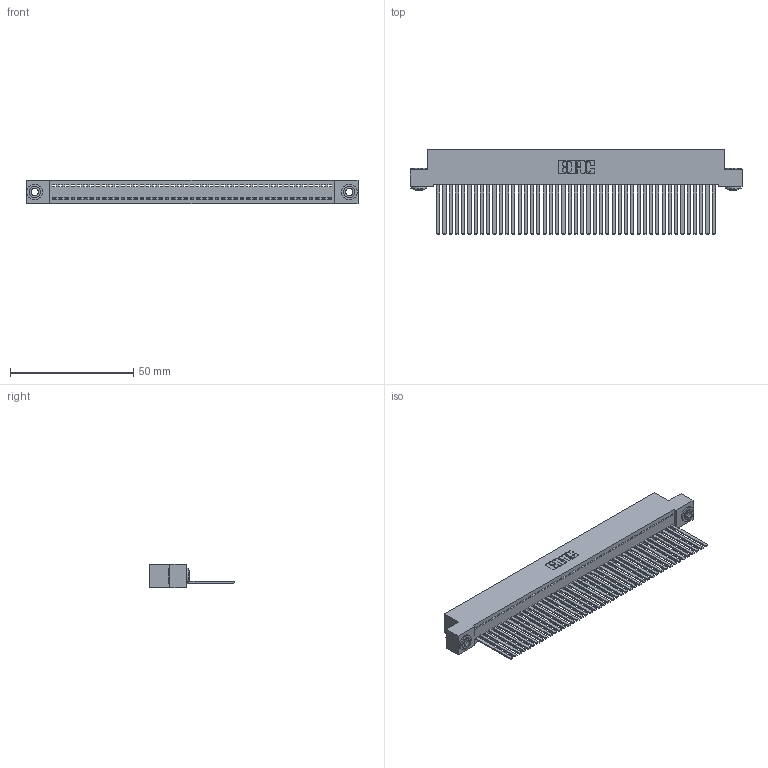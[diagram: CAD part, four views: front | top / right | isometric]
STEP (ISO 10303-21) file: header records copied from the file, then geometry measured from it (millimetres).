
FILE_DESCRIPTION (( 'STEP AP203' ), '1' );
FILE_NAME ('342-045-544-103.STEP', '2018-08-12T15:32:29', ( '' ), ( '' ), 'SwSTEP 2.0', 'SolidWorks 2016', '' );
FILE_SCHEMA (( 'CONFIG_CONTROL_DESIGN' ));
Length unit declared in the file: inch
Products named in the file (4): 342 Part_.156 TH; 345-292-001_345-293-144; 342-250-002_345-250-002-102; 342-045-544-103
Assembly tree (48 placements, depth 2):
  342-045-544-103
    342 Part_.156 TH
    345-292-001_345-293-144  x45
    342-250-002_345-250-002-102  x2
Bounding box: 134.62 x 34.3 x 9.4 mm (x, y, z)
Volume: 12358.5 mm3; surface area: 19913.4 mm2
Topology: 48 solids, 48 shells, 2488 faces, 7485 edges, 4926 vertices
Faces by surface type: plane 1786, cylinder 694, cone 8
Entity records: 27456 total; most frequent: CARTESIAN_POINT 4712, ORIENTED_EDGE 4686, DIRECTION 3999, EDGE_CURVE 2343, LINE 2195, VECTOR 2195, VERTEX_POINT 1558, AXIS2_PLACEMENT_3D 902
